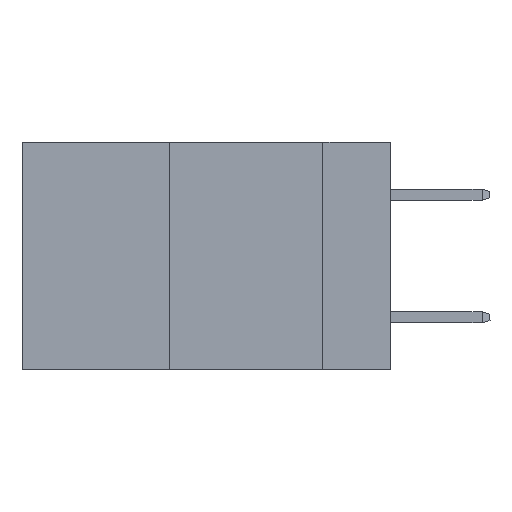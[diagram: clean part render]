
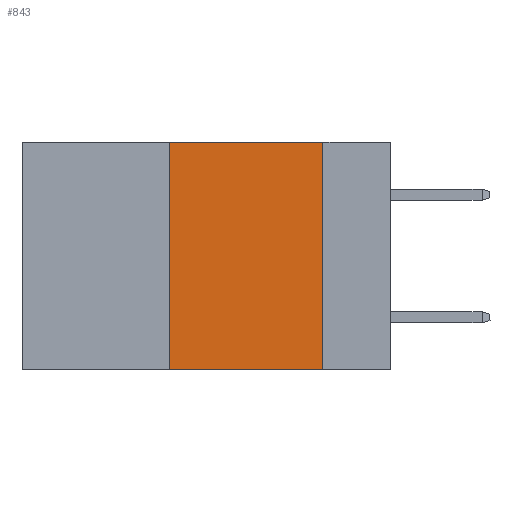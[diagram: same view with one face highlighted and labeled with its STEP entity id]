
A CAD part, left-side view. The second image highlights one B-rep face of the part: STEP entity #843.
In plain terms, the highlighted planar face has unit normal (-1, 0, 0).
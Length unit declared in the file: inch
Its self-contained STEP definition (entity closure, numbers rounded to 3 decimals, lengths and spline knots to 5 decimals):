
#275 = CARTESIAN_POINT ( 'NONE',  ( 0., 0.11, 0. ) ) ;
#449 = CARTESIAN_POINT ( 'NONE',  ( 0., 0.36, -0.37 ) ) ;
#843 = ADVANCED_FACE ( 'NONE', ( #14016 ), #8019, .F. ) ;
#1325 = VERTEX_POINT ( 'NONE', #10905 ) ;
#2751 = EDGE_CURVE ( 'NONE', #10960, #1325, #16854, .T. ) ;
#3050 = DIRECTION ( 'NONE',  ( 0., -1., 0. ) ) ;
#3352 = VECTOR ( 'NONE', #10989, 39.37008 ) ;
#4057 = ORIENTED_EDGE ( 'NONE', *, *, #12345, .T. ) ;
#5441 = VECTOR ( 'NONE', #19668, 39.37008 ) ;
#7381 = DIRECTION ( 'NONE',  ( 1., 0., 0. ) ) ;
#8019 = PLANE ( 'NONE',  #13905 ) ;
#9234 = EDGE_LOOP ( 'NONE', ( #10913, #18820, #11375, #4057 ) ) ;
#9253 = CARTESIAN_POINT ( 'NONE',  ( 0., 0.6, -0.37 ) ) ;
#9562 = DIRECTION ( 'NONE',  ( 0., 0., -1. ) ) ;
#10270 = VERTEX_POINT ( 'NONE', #449 ) ;
#10905 = CARTESIAN_POINT ( 'NONE',  ( 0., 0.11, 0. ) ) ;
#10913 = ORIENTED_EDGE ( 'NONE', *, *, #14317, .F. ) ;
#10960 = VERTEX_POINT ( 'NONE', #16163 ) ;
#10989 = DIRECTION ( 'NONE',  ( 0., 0., 1. ) ) ;
#11375 = ORIENTED_EDGE ( 'NONE', *, *, #14801, .F. ) ;
#11457 = DIRECTION ( 'NONE',  ( 0., 0., -1. ) ) ;
#12345 = EDGE_CURVE ( 'NONE', #10270, #12979, #13097, .T. ) ;
#12912 = VECTOR ( 'NONE', #3050, 39.37008 ) ;
#12979 = VERTEX_POINT ( 'NONE', #13791 ) ;
#13097 = LINE ( 'NONE', #9253, #5441 ) ;
#13791 = CARTESIAN_POINT ( 'NONE',  ( 0., 0.11, -0.37 ) ) ;
#13853 = CARTESIAN_POINT ( 'NONE',  ( 0., 0.6, 0. ) ) ;
#13905 = AXIS2_PLACEMENT_3D ( 'NONE', #19414, #7381, #9562 ) ;
#14016 = FACE_OUTER_BOUND ( 'NONE', #9234, .T. ) ;
#14317 = EDGE_CURVE ( 'NONE', #1325, #12979, #20023, .T. ) ;
#14801 = EDGE_CURVE ( 'NONE', #10270, #10960, #15104, .T. ) ;
#15104 = LINE ( 'NONE', #19881, #3352 ) ;
#16163 = CARTESIAN_POINT ( 'NONE',  ( 0., 0.36, 0. ) ) ;
#16517 = VECTOR ( 'NONE', #11457, 39.37008 ) ;
#16854 = LINE ( 'NONE', #13853, #12912 ) ;
#18820 = ORIENTED_EDGE ( 'NONE', *, *, #2751, .F. ) ;
#19414 = CARTESIAN_POINT ( 'NONE',  ( 0., 0.6, 0. ) ) ;
#19668 = DIRECTION ( 'NONE',  ( 0., -1., 0. ) ) ;
#19881 = CARTESIAN_POINT ( 'NONE',  ( 0., 0.36, 0. ) ) ;
#20023 = LINE ( 'NONE', #275, #16517 ) ;
